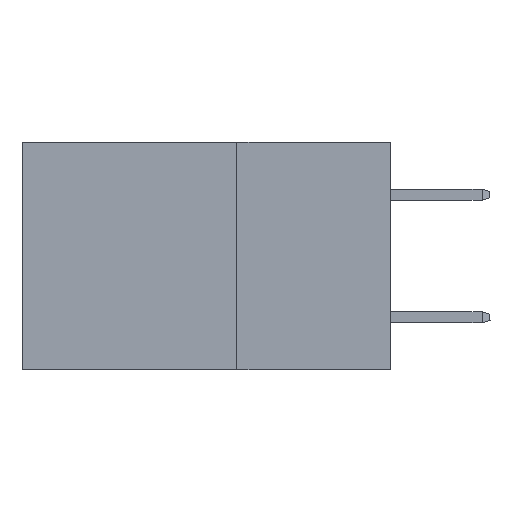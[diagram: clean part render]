
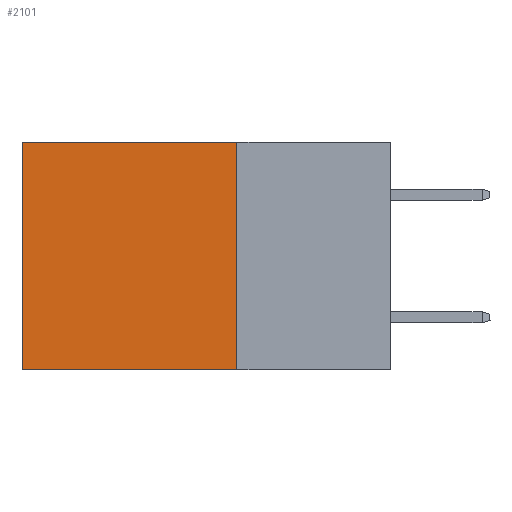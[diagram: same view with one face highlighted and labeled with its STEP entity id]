
A CAD part, left-side view. The second image highlights one B-rep face of the part: STEP entity #2101.
In plain terms, the highlighted planar face has unit normal (-1, 0, 0).
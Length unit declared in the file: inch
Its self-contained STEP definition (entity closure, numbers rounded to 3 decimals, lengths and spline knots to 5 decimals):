
#540 = CARTESIAN_POINT ( 'NONE',  ( 0.2875, 0.25, 0. ) ) ;
#2101 = ADVANCED_FACE ( 'NONE', ( #13693 ), #15921, .F. ) ;
#3035 = CARTESIAN_POINT ( 'NONE',  ( 0.2875, 0.25, 0. ) ) ;
#3116 = LINE ( 'NONE', #7534, #18346 ) ;
#4008 = DIRECTION ( 'NONE',  ( 0., 0., -1. ) ) ;
#5961 = DIRECTION ( 'NONE',  ( 1., 0., 0. ) ) ;
#7149 = DIRECTION ( 'NONE',  ( 0., 0., -1. ) ) ;
#7224 = VECTOR ( 'NONE', #18682, 39.37008 ) ;
#7523 = CARTESIAN_POINT ( 'NONE',  ( 0.2875, 0.6, 0. ) ) ;
#7534 = CARTESIAN_POINT ( 'NONE',  ( 0.2875, 0.25, 0. ) ) ;
#7835 = EDGE_LOOP ( 'NONE', ( #19823, #17248, #13320, #19132 ) ) ;
#9290 = EDGE_CURVE ( 'NONE', #11431, #9783, #3116, .T. ) ;
#9783 = VERTEX_POINT ( 'NONE', #7523 ) ;
#10773 = LINE ( 'NONE', #3035, #7224 ) ;
#11431 = VERTEX_POINT ( 'NONE', #540 ) ;
#11611 = VERTEX_POINT ( 'NONE', #22594 ) ;
#12076 = DIRECTION ( 'NONE',  ( 0., 1., 0. ) ) ;
#12354 = VECTOR ( 'NONE', #12076, 39.37008 ) ;
#13320 = ORIENTED_EDGE ( 'NONE', *, *, #29085, .F. ) ;
#13693 = FACE_OUTER_BOUND ( 'NONE', #7835, .T. ) ;
#14069 = CARTESIAN_POINT ( 'NONE',  ( 0.2875, 0.6, 0. ) ) ;
#14949 = CARTESIAN_POINT ( 'NONE',  ( 0.2875, 0.25, -0.37 ) ) ;
#15921 = PLANE ( 'NONE',  #26720 ) ;
#17248 = ORIENTED_EDGE ( 'NONE', *, *, #20045, .F. ) ;
#17681 = LINE ( 'NONE', #14069, #28915 ) ;
#18346 = VECTOR ( 'NONE', #25584, 39.37008 ) ;
#18682 = DIRECTION ( 'NONE',  ( 0., 0., -1. ) ) ;
#19132 = ORIENTED_EDGE ( 'NONE', *, *, #9290, .T. ) ;
#19306 = EDGE_CURVE ( 'NONE', #9783, #11611, #17681, .T. ) ;
#19823 = ORIENTED_EDGE ( 'NONE', *, *, #19306, .T. ) ;
#20045 = EDGE_CURVE ( 'NONE', #23749, #11611, #26771, .T. ) ;
#22594 = CARTESIAN_POINT ( 'NONE',  ( 0.2875, 0.6, -0.37 ) ) ;
#23749 = VERTEX_POINT ( 'NONE', #14949 ) ;
#24842 = CARTESIAN_POINT ( 'NONE',  ( 0.2875, 0.25, 0. ) ) ;
#25584 = DIRECTION ( 'NONE',  ( 0., 1., 0. ) ) ;
#26720 = AXIS2_PLACEMENT_3D ( 'NONE', #24842, #5961, #4008 ) ;
#26771 = LINE ( 'NONE', #27734, #12354 ) ;
#27734 = CARTESIAN_POINT ( 'NONE',  ( 0.2875, 0.25, -0.37 ) ) ;
#28915 = VECTOR ( 'NONE', #7149, 39.37008 ) ;
#29085 = EDGE_CURVE ( 'NONE', #11431, #23749, #10773, .T. ) ;
